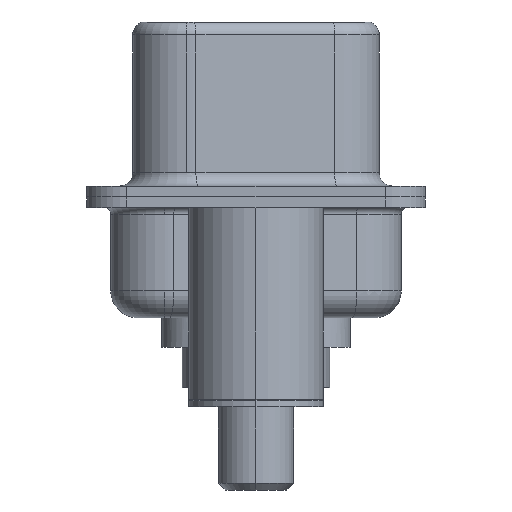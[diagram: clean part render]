
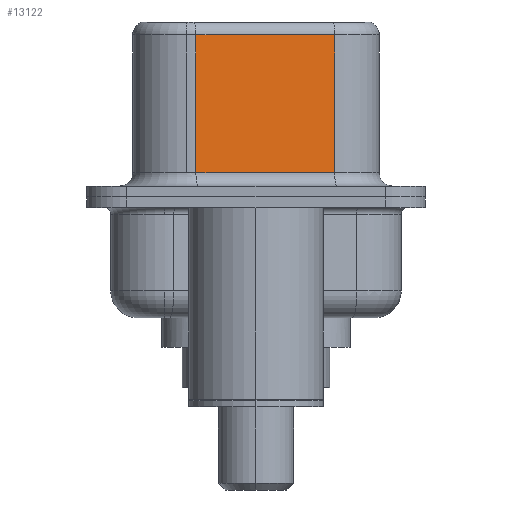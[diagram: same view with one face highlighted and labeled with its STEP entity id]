
A CAD part, left-side view. The second image highlights one B-rep face of the part: STEP entity #13122.
In plain terms, the highlighted planar face has unit normal (-0.985, -0.174, 0).
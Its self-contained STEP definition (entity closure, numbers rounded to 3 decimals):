
#189 = AXIS2_PLACEMENT_3D ( 'NONE', #4145, #12092, #5335 ) ;
#439 = CARTESIAN_POINT ( 'NONE',  ( 4.58, -2.927, 6.02 ) ) ;
#775 = EDGE_LOOP ( 'NONE', ( #10870, #5916, #5463, #1913 ) ) ;
#1691 = VECTOR ( 'NONE', #2801, 1000. ) ;
#1913 = ORIENTED_EDGE ( 'NONE', *, *, #13071, .T. ) ;
#2042 = LINE ( 'NONE', #7579, #1691 ) ;
#2306 = DIRECTION ( 'NONE',  ( 0., 0., -1. ) ) ;
#2610 = VERTEX_POINT ( 'NONE', #439 ) ;
#2801 = DIRECTION ( 'NONE',  ( 0.174, -0.985, 0. ) ) ;
#3792 = VERTEX_POINT ( 'NONE', #13777 ) ;
#4145 = CARTESIAN_POINT ( 'NONE',  ( 4.58, -2.927, 6.52 ) ) ;
#4223 = VERTEX_POINT ( 'NONE', #11943 ) ;
#5317 = VECTOR ( 'NONE', #7286, 1000. ) ;
#5335 = DIRECTION ( 'NONE',  ( -0.174, 0.985, 0. ) ) ;
#5463 = ORIENTED_EDGE ( 'NONE', *, *, #7725, .T. ) ;
#5527 = VECTOR ( 'NONE', #2306, 1000. ) ;
#5885 = LINE ( 'NONE', #9308, #5527 ) ;
#5916 = ORIENTED_EDGE ( 'NONE', *, *, #8722, .T. ) ;
#5961 = CARTESIAN_POINT ( 'NONE',  ( 4.58, -2.927, 6.52 ) ) ;
#7286 = DIRECTION ( 'NONE',  ( -0.174, 0.985, 0. ) ) ;
#7296 = VERTEX_POINT ( 'NONE', #14151 ) ;
#7574 = VECTOR ( 'NONE', #12710, 1000. ) ;
#7579 = CARTESIAN_POINT ( 'NONE',  ( 4.58, -2.927, 0.9 ) ) ;
#7725 = EDGE_CURVE ( 'NONE', #7296, #4223, #5885, .T. ) ;
#8359 = LINE ( 'NONE', #10621, #5317 ) ;
#8722 = EDGE_CURVE ( 'NONE', #2610, #7296, #8359, .T. ) ;
#8730 = PLANE ( 'NONE',  #189 ) ;
#9308 = CARTESIAN_POINT ( 'NONE',  ( 3.67, 2.233, 6.52 ) ) ;
#10621 = CARTESIAN_POINT ( 'NONE',  ( 4.58, -2.927, 6.02 ) ) ;
#10870 = ORIENTED_EDGE ( 'NONE', *, *, #14027, .F. ) ;
#11943 = CARTESIAN_POINT ( 'NONE',  ( 3.67, 2.233, 0.9 ) ) ;
#12092 = DIRECTION ( 'NONE',  ( 0.985, 0.174, 0. ) ) ;
#12710 = DIRECTION ( 'NONE',  ( 0., 0., -1. ) ) ;
#13071 = EDGE_CURVE ( 'NONE', #4223, #3792, #2042, .T. ) ;
#13122 = ADVANCED_FACE ( 'NONE', ( #13539 ), #8730, .F. ) ;
#13539 = FACE_OUTER_BOUND ( 'NONE', #775, .T. ) ;
#13777 = CARTESIAN_POINT ( 'NONE',  ( 4.58, -2.927, 0.9 ) ) ;
#13874 = LINE ( 'NONE', #5961, #7574 ) ;
#14027 = EDGE_CURVE ( 'NONE', #2610, #3792, #13874, .T. ) ;
#14151 = CARTESIAN_POINT ( 'NONE',  ( 3.67, 2.233, 6.02 ) ) ;
